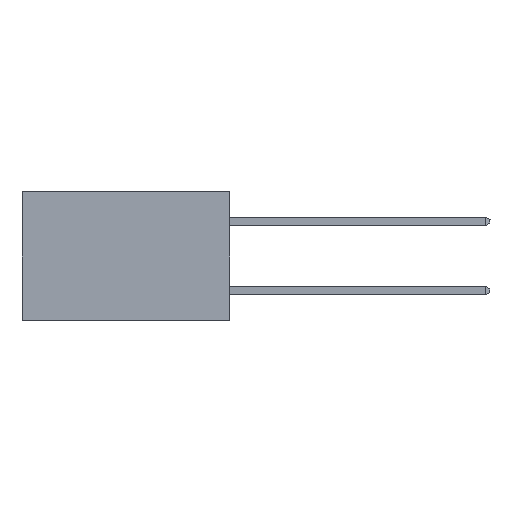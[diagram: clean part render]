
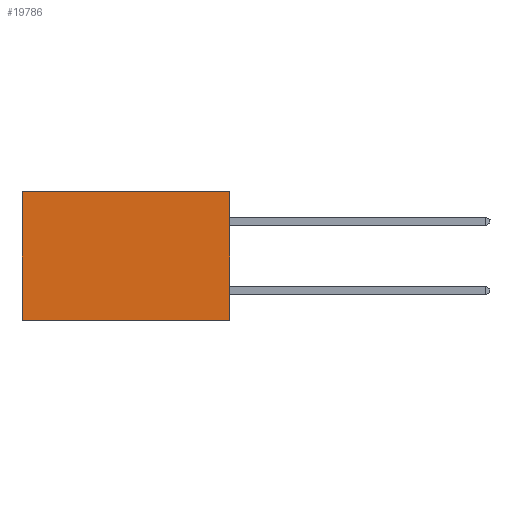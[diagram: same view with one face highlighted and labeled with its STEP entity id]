
A CAD part, left-side view. The second image highlights one B-rep face of the part: STEP entity #19786.
In plain terms, the highlighted planar face has unit normal (-1, 0, 0).
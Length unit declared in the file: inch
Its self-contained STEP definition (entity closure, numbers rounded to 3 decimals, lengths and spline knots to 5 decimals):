
#444 = CARTESIAN_POINT ( 'NONE',  ( 0.2615, 0.6, -0.37 ) ) ;
#463 = CARTESIAN_POINT ( 'NONE',  ( 0.2615, 0., -0.37 ) ) ;
#1856 = EDGE_CURVE ( 'NONE', #9021, #10566, #4447, .T. ) ;
#2661 = CARTESIAN_POINT ( 'NONE',  ( 0.2615, 0.6, 0. ) ) ;
#3710 = AXIS2_PLACEMENT_3D ( 'NONE', #7032, #19917, #16379 ) ;
#4447 = LINE ( 'NONE', #18778, #14454 ) ;
#5367 = LINE ( 'NONE', #10262, #6846 ) ;
#5733 = DIRECTION ( 'NONE',  ( 0., 1., 0. ) ) ;
#6447 = ORIENTED_EDGE ( 'NONE', *, *, #13568, .T. ) ;
#6846 = VECTOR ( 'NONE', #11426, 39.37008 ) ;
#7032 = CARTESIAN_POINT ( 'NONE',  ( 0.2615, 0., -0.37 ) ) ;
#8980 = ORIENTED_EDGE ( 'NONE', *, *, #11890, .T. ) ;
#9021 = VERTEX_POINT ( 'NONE', #463 ) ;
#10262 = CARTESIAN_POINT ( 'NONE',  ( 0.2615, 0.6, -0.37 ) ) ;
#10394 = EDGE_LOOP ( 'NONE', ( #8980, #11335, #11392, #6447 ) ) ;
#10566 = VERTEX_POINT ( 'NONE', #444 ) ;
#10845 = LINE ( 'NONE', #17261, #13948 ) ;
#11335 = ORIENTED_EDGE ( 'NONE', *, *, #1856, .F. ) ;
#11392 = ORIENTED_EDGE ( 'NONE', *, *, #13823, .F. ) ;
#11426 = DIRECTION ( 'NONE',  ( 0., 0., -1. ) ) ;
#11595 = VECTOR ( 'NONE', #15213, 39.37008 ) ;
#11747 = PLANE ( 'NONE',  #3710 ) ;
#11890 = EDGE_CURVE ( 'NONE', #18704, #10566, #5367, .T. ) ;
#12155 = LINE ( 'NONE', #16997, #11595 ) ;
#12160 = VERTEX_POINT ( 'NONE', #17681 ) ;
#13568 = EDGE_CURVE ( 'NONE', #12160, #18704, #10845, .T. ) ;
#13823 = EDGE_CURVE ( 'NONE', #12160, #9021, #12155, .T. ) ;
#13948 = VECTOR ( 'NONE', #5733, 39.37008 ) ;
#14454 = VECTOR ( 'NONE', #17212, 39.37008 ) ;
#15213 = DIRECTION ( 'NONE',  ( 0., 0., -1. ) ) ;
#16379 = DIRECTION ( 'NONE',  ( 0., 0., -1. ) ) ;
#16997 = CARTESIAN_POINT ( 'NONE',  ( 0.2615, 0., -0.37 ) ) ;
#17212 = DIRECTION ( 'NONE',  ( 0., 1., 0. ) ) ;
#17261 = CARTESIAN_POINT ( 'NONE',  ( 0.2615, 0., 0. ) ) ;
#17681 = CARTESIAN_POINT ( 'NONE',  ( 0.2615, 0., 0. ) ) ;
#18704 = VERTEX_POINT ( 'NONE', #2661 ) ;
#18778 = CARTESIAN_POINT ( 'NONE',  ( 0.2615, 0., -0.37 ) ) ;
#19505 = FACE_OUTER_BOUND ( 'NONE', #10394, .T. ) ;
#19786 = ADVANCED_FACE ( 'NONE', ( #19505 ), #11747, .F. ) ;
#19917 = DIRECTION ( 'NONE',  ( 1., 0., 0. ) ) ;
